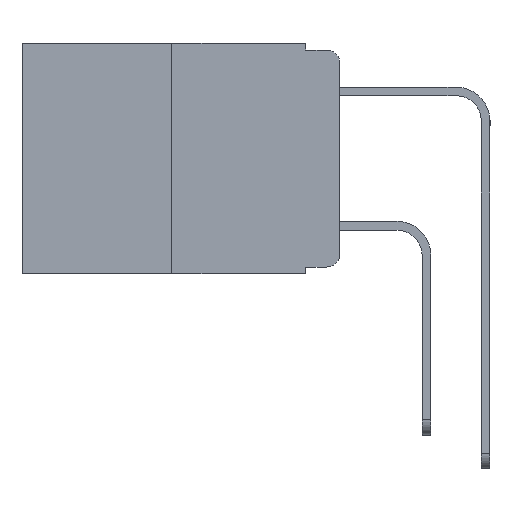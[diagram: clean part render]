
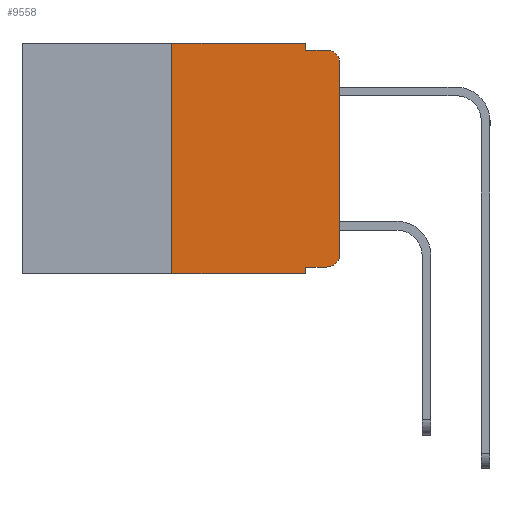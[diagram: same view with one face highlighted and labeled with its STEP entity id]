
A CAD part, left-side view. The second image highlights one B-rep face of the part: STEP entity #9558.
In plain terms, the highlighted planar face has unit normal (-1, 0, 0).
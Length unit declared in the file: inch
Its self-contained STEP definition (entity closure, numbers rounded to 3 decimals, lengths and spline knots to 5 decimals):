
#426 = VERTEX_POINT ( 'NONE', #11410 ) ;
#432 = VECTOR ( 'NONE', #989, 39.37008 ) ;
#989 = DIRECTION ( 'NONE',  ( 0., 0., -1. ) ) ;
#1086 = CARTESIAN_POINT ( 'NONE',  ( 0., 0.02, -0.03 ) ) ;
#1120 = CARTESIAN_POINT ( 'NONE',  ( 0., 0.051, 0. ) ) ;
#1510 = ORIENTED_EDGE ( 'NONE', *, *, #4987, .F. ) ;
#1659 = LINE ( 'NONE', #15626, #14338 ) ;
#1970 = ORIENTED_EDGE ( 'NONE', *, *, #5790, .F. ) ;
#1974 = CARTESIAN_POINT ( 'NONE',  ( 0., 0.473, 0. ) ) ;
#2275 = EDGE_CURVE ( 'NONE', #13499, #3556, #11083, .T. ) ;
#2416 = ORIENTED_EDGE ( 'NONE', *, *, #7424, .T. ) ;
#2529 = DIRECTION ( 'NONE',  ( 0., 0., -1. ) ) ;
#2558 = AXIS2_PLACEMENT_3D ( 'NONE', #5788, #5768, #5744 ) ;
#3265 = EDGE_CURVE ( 'NONE', #13275, #13499, #12521, .T. ) ;
#3303 = CARTESIAN_POINT ( 'NONE',  ( 0., 0.051, 0. ) ) ;
#3556 = VERTEX_POINT ( 'NONE', #15114 ) ;
#3870 = VERTEX_POINT ( 'NONE', #12841 ) ;
#3925 = DIRECTION ( 'NONE',  ( 0., 0., 1. ) ) ;
#4031 = CARTESIAN_POINT ( 'NONE',  ( 0., 0.02, -0.333 ) ) ;
#4189 = EDGE_CURVE ( 'NONE', #13275, #14583, #10622, .T. ) ;
#4313 = CARTESIAN_POINT ( 'NONE',  ( 0., 0.25, -0.343 ) ) ;
#4893 = EDGE_CURVE ( 'NONE', #3870, #12150, #12460, .T. ) ;
#4954 = ORIENTED_EDGE ( 'NONE', *, *, #3265, .T. ) ;
#4963 = VECTOR ( 'NONE', #5988, 39.37008 ) ;
#4987 = EDGE_CURVE ( 'NONE', #8386, #3870, #14753, .T. ) ;
#5354 = PLANE ( 'NONE',  #8461 ) ;
#5697 = VECTOR ( 'NONE', #11800, 39.37008 ) ;
#5744 = DIRECTION ( 'NONE',  ( 0., 0., -1. ) ) ;
#5768 = DIRECTION ( 'NONE',  ( -1., 0., 0. ) ) ;
#5788 = CARTESIAN_POINT ( 'NONE',  ( 0., 0.02, -0.313 ) ) ;
#5790 = EDGE_CURVE ( 'NONE', #12150, #9328, #15732, .T. ) ;
#5988 = DIRECTION ( 'NONE',  ( 0., 0., 1. ) ) ;
#6091 = VECTOR ( 'NONE', #11928, 39.37008 ) ;
#6150 = VECTOR ( 'NONE', #12818, 39.37008 ) ;
#6565 = CARTESIAN_POINT ( 'NONE',  ( 0., 0.473, 0. ) ) ;
#6588 = EDGE_CURVE ( 'NONE', #9328, #12207, #11131, .T. ) ;
#6880 = CARTESIAN_POINT ( 'NONE',  ( 0., 0.051, -0.333 ) ) ;
#7264 = CARTESIAN_POINT ( 'NONE',  ( 0., 0.25, 0. ) ) ;
#7362 = EDGE_LOOP ( 'NONE', ( #12276, #2416, #11900, #1970, #11505, #1510, #14220, #7946, #4954, #7776 ) ) ;
#7424 = EDGE_CURVE ( 'NONE', #426, #12207, #13112, .T. ) ;
#7776 = ORIENTED_EDGE ( 'NONE', *, *, #2275, .T. ) ;
#7781 = DIRECTION ( 'NONE',  ( 0., 0., -1. ) ) ;
#7803 = VECTOR ( 'NONE', #8966, 39.37008 ) ;
#7946 = ORIENTED_EDGE ( 'NONE', *, *, #4189, .F. ) ;
#8208 = EDGE_CURVE ( 'NONE', #3556, #426, #1659, .T. ) ;
#8386 = VERTEX_POINT ( 'NONE', #4313 ) ;
#8461 = AXIS2_PLACEMENT_3D ( 'NONE', #6565, #14803, #7781 ) ;
#8716 = CARTESIAN_POINT ( 'NONE',  ( 0., 0.051, 0. ) ) ;
#8910 = CARTESIAN_POINT ( 'NONE',  ( 0., 0.473, -0.343 ) ) ;
#8966 = DIRECTION ( 'NONE',  ( 0., -1., 0. ) ) ;
#9328 = VERTEX_POINT ( 'NONE', #9478 ) ;
#9478 = CARTESIAN_POINT ( 'NONE',  ( 0., 0.051, -0.01 ) ) ;
#9530 = EDGE_CURVE ( 'NONE', #8386, #14583, #11007, .T. ) ;
#9558 = ADVANCED_FACE ( 'NONE', ( #13712 ), #5354, .F. ) ;
#9869 = CARTESIAN_POINT ( 'NONE',  ( 0., 0.051, -0.01 ) ) ;
#10000 = DIRECTION ( 'NONE',  ( -1., 0., 0. ) ) ;
#10317 = AXIS2_PLACEMENT_3D ( 'NONE', #1086, #10000, #2529 ) ;
#10418 = CARTESIAN_POINT ( 'NONE',  ( 0., 0.051, -0.343 ) ) ;
#10622 = LINE ( 'NONE', #8716, #432 ) ;
#10766 = VECTOR ( 'NONE', #14490, 39.37008 ) ;
#11007 = LINE ( 'NONE', #8910, #7803 ) ;
#11083 = CIRCLE ( 'NONE', #2558, 0.02 ) ;
#11131 = LINE ( 'NONE', #9869, #10766 ) ;
#11410 = CARTESIAN_POINT ( 'NONE',  ( 0., 0., -0.03 ) ) ;
#11505 = ORIENTED_EDGE ( 'NONE', *, *, #4893, .F. ) ;
#11800 = DIRECTION ( 'NONE',  ( 0., 0., -1. ) ) ;
#11900 = ORIENTED_EDGE ( 'NONE', *, *, #6588, .F. ) ;
#11928 = DIRECTION ( 'NONE',  ( 0., -1., 0. ) ) ;
#12150 = VERTEX_POINT ( 'NONE', #1120 ) ;
#12207 = VERTEX_POINT ( 'NONE', #13596 ) ;
#12276 = ORIENTED_EDGE ( 'NONE', *, *, #8208, .T. ) ;
#12460 = LINE ( 'NONE', #1974, #6091 ) ;
#12521 = LINE ( 'NONE', #6880, #6150 ) ;
#12818 = DIRECTION ( 'NONE',  ( 0., -1., 0. ) ) ;
#12841 = CARTESIAN_POINT ( 'NONE',  ( 0., 0.25, 0. ) ) ;
#13059 = CARTESIAN_POINT ( 'NONE',  ( 0., 0.051, -0.333 ) ) ;
#13112 = CIRCLE ( 'NONE', #10317, 0.02 ) ;
#13275 = VERTEX_POINT ( 'NONE', #13059 ) ;
#13499 = VERTEX_POINT ( 'NONE', #4031 ) ;
#13596 = CARTESIAN_POINT ( 'NONE',  ( 0., 0.02, -0.01 ) ) ;
#13712 = FACE_OUTER_BOUND ( 'NONE', #7362, .T. ) ;
#14220 = ORIENTED_EDGE ( 'NONE', *, *, #9530, .T. ) ;
#14338 = VECTOR ( 'NONE', #3925, 39.37008 ) ;
#14490 = DIRECTION ( 'NONE',  ( 0., -1., 0. ) ) ;
#14583 = VERTEX_POINT ( 'NONE', #10418 ) ;
#14753 = LINE ( 'NONE', #7264, #4963 ) ;
#14803 = DIRECTION ( 'NONE',  ( 1., 0., 0. ) ) ;
#15114 = CARTESIAN_POINT ( 'NONE',  ( 0., 0., -0.313 ) ) ;
#15626 = CARTESIAN_POINT ( 'NONE',  ( 0., 0., 0. ) ) ;
#15732 = LINE ( 'NONE', #3303, #5697 ) ;
